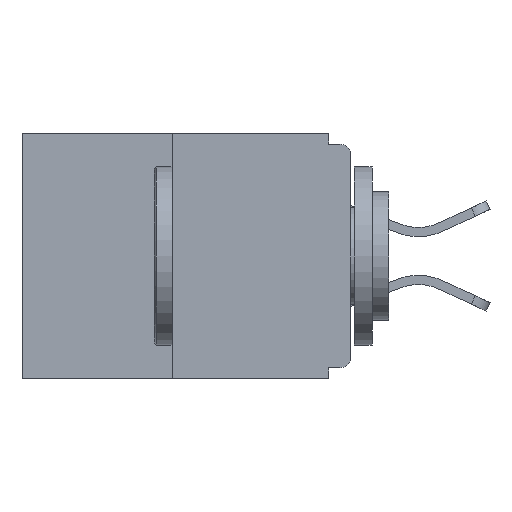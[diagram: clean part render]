
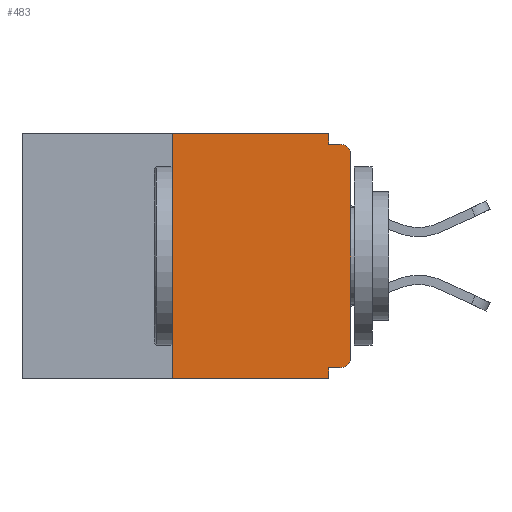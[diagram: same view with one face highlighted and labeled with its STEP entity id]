
A CAD part, left-side view. The second image highlights one B-rep face of the part: STEP entity #483.
In plain terms, the highlighted planar face has unit normal (-1, 0, 0).
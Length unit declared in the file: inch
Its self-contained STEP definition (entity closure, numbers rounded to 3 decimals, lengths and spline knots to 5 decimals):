
#100 = EDGE_CURVE ( 'NONE', #21974, #17136, #4268, .T. ) ;
#483 = ADVANCED_FACE ( 'NONE', ( #23320 ), #4125, .F. ) ;
#706 = EDGE_CURVE ( 'NONE', #21885, #4505, #21786, .T. ) ;
#800 = AXIS2_PLACEMENT_3D ( 'NONE', #31875, #19737, #12127 ) ;
#1026 = VERTEX_POINT ( 'NONE', #19848 ) ;
#1310 = ORIENTED_EDGE ( 'NONE', *, *, #6949, .F. ) ;
#1715 = DIRECTION ( 'NONE',  ( 1., 0., 0. ) ) ;
#2532 = EDGE_CURVE ( 'NONE', #6978, #15000, #8257, .T. ) ;
#2539 = LINE ( 'NONE', #31246, #29057 ) ;
#2586 = LINE ( 'NONE', #21271, #3757 ) ;
#3203 = VERTEX_POINT ( 'NONE', #27276 ) ;
#3433 = DIRECTION ( 'NONE',  ( -1., 0., 0. ) ) ;
#3757 = VECTOR ( 'NONE', #23445, 39.37008 ) ;
#4125 = PLANE ( 'NONE',  #24931 ) ;
#4268 = LINE ( 'NONE', #4776, #23355 ) ;
#4505 = VERTEX_POINT ( 'NONE', #25732 ) ;
#4776 = CARTESIAN_POINT ( 'NONE',  ( 0., 0.46, 0. ) ) ;
#5386 = VECTOR ( 'NONE', #15933, 39.37008 ) ;
#5949 = DIRECTION ( 'NONE',  ( 0., 0., -1. ) ) ;
#6330 = VECTOR ( 'NONE', #12194, 39.37008 ) ;
#6949 = EDGE_CURVE ( 'NONE', #3203, #21974, #2539, .T. ) ;
#6978 = VERTEX_POINT ( 'NONE', #21200 ) ;
#6987 = CARTESIAN_POINT ( 'NONE',  ( 0., 0., -0.015 ) ) ;
#7825 = CIRCLE ( 'NONE', #800, 0.015 ) ;
#7982 = CARTESIAN_POINT ( 'NONE',  ( 0., 0.031, -0.328 ) ) ;
#8193 = CARTESIAN_POINT ( 'NONE',  ( 0., 0., 0. ) ) ;
#8257 = LINE ( 'NONE', #22091, #6330 ) ;
#9138 = CARTESIAN_POINT ( 'NONE',  ( 0., 0.46, 0. ) ) ;
#9331 = VECTOR ( 'NONE', #26452, 39.37008 ) ;
#10061 = LINE ( 'NONE', #6987, #27243 ) ;
#11385 = ORIENTED_EDGE ( 'NONE', *, *, #706, .T. ) ;
#11901 = ORIENTED_EDGE ( 'NONE', *, *, #29091, .T. ) ;
#12127 = DIRECTION ( 'NONE',  ( 0., 0., -1. ) ) ;
#12194 = DIRECTION ( 'NONE',  ( 0., 1., 0. ) ) ;
#13399 = VERTEX_POINT ( 'NONE', #22148 ) ;
#14816 = CARTESIAN_POINT ( 'NONE',  ( 0., 0., -0.313 ) ) ;
#15000 = VERTEX_POINT ( 'NONE', #7982 ) ;
#15097 = VERTEX_POINT ( 'NONE', #28920 ) ;
#15455 = CARTESIAN_POINT ( 'NONE',  ( 0., 0.25, 0. ) ) ;
#15933 = DIRECTION ( 'NONE',  ( 0., 0., 1. ) ) ;
#15944 = LINE ( 'NONE', #27228, #9331 ) ;
#16203 = CARTESIAN_POINT ( 'NONE',  ( 0., 0.015, -0.03 ) ) ;
#17131 = ORIENTED_EDGE ( 'NONE', *, *, #22368, .F. ) ;
#17136 = VERTEX_POINT ( 'NONE', #31101 ) ;
#17422 = DIRECTION ( 'NONE',  ( 0., -1., 0. ) ) ;
#17930 = LINE ( 'NONE', #29664, #30647 ) ;
#18394 = DIRECTION ( 'NONE',  ( 0., 0., -1. ) ) ;
#19242 = ORIENTED_EDGE ( 'NONE', *, *, #100, .F. ) ;
#19333 = ORIENTED_EDGE ( 'NONE', *, *, #20092, .F. ) ;
#19733 = DIRECTION ( 'NONE',  ( 0., 0., -1. ) ) ;
#19737 = DIRECTION ( 'NONE',  ( -1., 0., 0. ) ) ;
#19848 = CARTESIAN_POINT ( 'NONE',  ( 0., 0.015, -0.015 ) ) ;
#19986 = EDGE_CURVE ( 'NONE', #13399, #1026, #10061, .T. ) ;
#20092 = EDGE_CURVE ( 'NONE', #15000, #15097, #17930, .T. ) ;
#20503 = ORIENTED_EDGE ( 'NONE', *, *, #28611, .T. ) ;
#21200 = CARTESIAN_POINT ( 'NONE',  ( 0., 0.015, -0.328 ) ) ;
#21271 = CARTESIAN_POINT ( 'NONE',  ( 0., 0.46, -0.343 ) ) ;
#21588 = EDGE_LOOP ( 'NONE', ( #19242, #1310, #20503, #19333, #32015, #22989, #11385, #11901, #25271, #17131 ) ) ;
#21786 = LINE ( 'NONE', #8193, #5386 ) ;
#21885 = VERTEX_POINT ( 'NONE', #14816 ) ;
#21974 = VERTEX_POINT ( 'NONE', #15455 ) ;
#22091 = CARTESIAN_POINT ( 'NONE',  ( 0., 0., -0.328 ) ) ;
#22148 = CARTESIAN_POINT ( 'NONE',  ( 0., 0.031, -0.015 ) ) ;
#22368 = EDGE_CURVE ( 'NONE', #17136, #13399, #15944, .T. ) ;
#22989 = ORIENTED_EDGE ( 'NONE', *, *, #31746, .T. ) ;
#23281 = AXIS2_PLACEMENT_3D ( 'NONE', #16203, #3433, #5949 ) ;
#23320 = FACE_OUTER_BOUND ( 'NONE', #21588, .T. ) ;
#23355 = VECTOR ( 'NONE', #17422, 39.37008 ) ;
#23445 = DIRECTION ( 'NONE',  ( 0., -1., 0. ) ) ;
#23604 = CIRCLE ( 'NONE', #23281, 0.015 ) ;
#24931 = AXIS2_PLACEMENT_3D ( 'NONE', #9138, #1715, #18394 ) ;
#25271 = ORIENTED_EDGE ( 'NONE', *, *, #19986, .F. ) ;
#25732 = CARTESIAN_POINT ( 'NONE',  ( 0., 0., -0.03 ) ) ;
#26452 = DIRECTION ( 'NONE',  ( 0., 0., -1. ) ) ;
#26473 = DIRECTION ( 'NONE',  ( 0., 0., 1. ) ) ;
#26986 = DIRECTION ( 'NONE',  ( 0., -1., 0. ) ) ;
#27228 = CARTESIAN_POINT ( 'NONE',  ( 0., 0.031, 0. ) ) ;
#27243 = VECTOR ( 'NONE', #26986, 39.37008 ) ;
#27276 = CARTESIAN_POINT ( 'NONE',  ( 0., 0.25, -0.343 ) ) ;
#28611 = EDGE_CURVE ( 'NONE', #3203, #15097, #2586, .T. ) ;
#28920 = CARTESIAN_POINT ( 'NONE',  ( 0., 0.031, -0.343 ) ) ;
#29057 = VECTOR ( 'NONE', #26473, 39.37008 ) ;
#29091 = EDGE_CURVE ( 'NONE', #4505, #1026, #23604, .T. ) ;
#29664 = CARTESIAN_POINT ( 'NONE',  ( 0., 0.031, -0.343 ) ) ;
#30647 = VECTOR ( 'NONE', #19733, 39.37008 ) ;
#31101 = CARTESIAN_POINT ( 'NONE',  ( 0., 0.031, 0. ) ) ;
#31246 = CARTESIAN_POINT ( 'NONE',  ( 0., 0.25, 0. ) ) ;
#31746 = EDGE_CURVE ( 'NONE', #6978, #21885, #7825, .T. ) ;
#31875 = CARTESIAN_POINT ( 'NONE',  ( 0., 0.015, -0.313 ) ) ;
#32015 = ORIENTED_EDGE ( 'NONE', *, *, #2532, .F. ) ;
